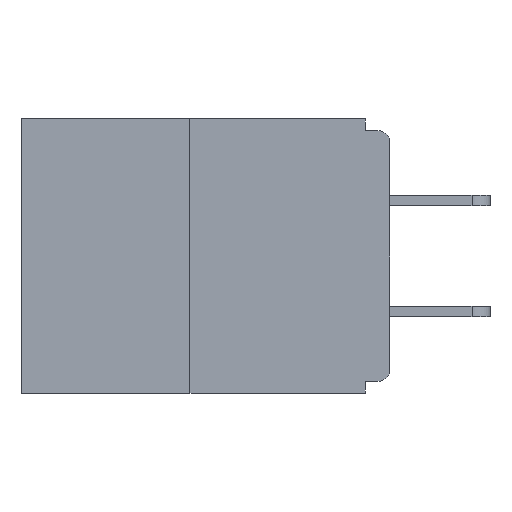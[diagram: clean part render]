
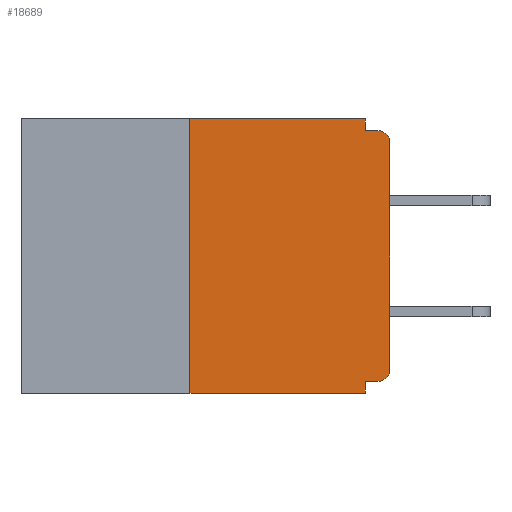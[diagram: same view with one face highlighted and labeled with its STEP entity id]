
A CAD part, left-side view. The second image highlights one B-rep face of the part: STEP entity #18689.
In plain terms, the highlighted planar face has unit normal (-1, 0, 0).
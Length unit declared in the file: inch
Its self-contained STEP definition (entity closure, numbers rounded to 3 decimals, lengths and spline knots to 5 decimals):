
#1026 = VERTEX_POINT ( 'NONE', #18729 ) ;
#1028 = CARTESIAN_POINT ( 'NONE',  ( 0., 0.46, 0. ) ) ;
#1231 = EDGE_CURVE ( 'NONE', #10391, #13205, #14252, .T. ) ;
#1282 = CARTESIAN_POINT ( 'NONE',  ( 0., 0.031, 0. ) ) ;
#1379 = EDGE_LOOP ( 'NONE', ( #12505, #6901, #14425, #8585, #7923, #14667, #17898, #1803, #16608, #10620 ) ) ;
#1416 = CARTESIAN_POINT ( 'NONE',  ( 0., 0., -0.015 ) ) ;
#1549 = CIRCLE ( 'NONE', #18769, 0.015 ) ;
#1803 = ORIENTED_EDGE ( 'NONE', *, *, #17479, .T. ) ;
#2152 = VECTOR ( 'NONE', #8442, 39.37008 ) ;
#2327 = CARTESIAN_POINT ( 'NONE',  ( 0., 0.031, -0.328 ) ) ;
#3012 = DIRECTION ( 'NONE',  ( 0., 0., -1. ) ) ;
#3296 = DIRECTION ( 'NONE',  ( 0., 1., 0. ) ) ;
#3542 = EDGE_CURVE ( 'NONE', #10391, #17923, #11056, .T. ) ;
#3973 = CARTESIAN_POINT ( 'NONE',  ( 0., 0.015, -0.313 ) ) ;
#4038 = DIRECTION ( 'NONE',  ( 0., 0., -1. ) ) ;
#4363 = LINE ( 'NONE', #1028, #18585 ) ;
#5464 = DIRECTION ( 'NONE',  ( 0., -1., 0. ) ) ;
#5690 = EDGE_CURVE ( 'NONE', #8635, #8324, #1549, .T. ) ;
#6554 = CARTESIAN_POINT ( 'NONE',  ( 0., 0.015, -0.03 ) ) ;
#6901 = ORIENTED_EDGE ( 'NONE', *, *, #3542, .F. ) ;
#6946 = DIRECTION ( 'NONE',  ( 0., 0., 1. ) ) ;
#7011 = CARTESIAN_POINT ( 'NONE',  ( 0., 0.25, 0. ) ) ;
#7147 = EDGE_CURVE ( 'NONE', #17923, #12711, #4363, .T. ) ;
#7442 = PLANE ( 'NONE',  #8067 ) ;
#7923 = ORIENTED_EDGE ( 'NONE', *, *, #11989, .F. ) ;
#8022 = DIRECTION ( 'NONE',  ( 0., 0., -1. ) ) ;
#8067 = AXIS2_PLACEMENT_3D ( 'NONE', #11747, #15289, #3012 ) ;
#8088 = LINE ( 'NONE', #19436, #18518 ) ;
#8324 = VERTEX_POINT ( 'NONE', #12617 ) ;
#8442 = DIRECTION ( 'NONE',  ( 0., -1., 0. ) ) ;
#8585 = ORIENTED_EDGE ( 'NONE', *, *, #10403, .F. ) ;
#8635 = VERTEX_POINT ( 'NONE', #10607 ) ;
#9167 = CARTESIAN_POINT ( 'NONE',  ( 0., 0.25, 0. ) ) ;
#9355 = VECTOR ( 'NONE', #3296, 39.37008 ) ;
#10145 = LINE ( 'NONE', #1282, #10378 ) ;
#10183 = EDGE_CURVE ( 'NONE', #12711, #17904, #10145, .T. ) ;
#10360 = VERTEX_POINT ( 'NONE', #2327 ) ;
#10378 = VECTOR ( 'NONE', #11878, 39.37008 ) ;
#10391 = VERTEX_POINT ( 'NONE', #18839 ) ;
#10403 = EDGE_CURVE ( 'NONE', #10360, #13205, #13717, .T. ) ;
#10540 = LINE ( 'NONE', #10839, #9355 ) ;
#10607 = CARTESIAN_POINT ( 'NONE',  ( 0., 0.015, -0.328 ) ) ;
#10620 = ORIENTED_EDGE ( 'NONE', *, *, #10183, .F. ) ;
#10839 = CARTESIAN_POINT ( 'NONE',  ( 0., 0., -0.328 ) ) ;
#11056 = LINE ( 'NONE', #7011, #18648 ) ;
#11747 = CARTESIAN_POINT ( 'NONE',  ( 0., 0.46, 0. ) ) ;
#11878 = DIRECTION ( 'NONE',  ( 0., 0., -1. ) ) ;
#11989 = EDGE_CURVE ( 'NONE', #8635, #10360, #10540, .T. ) ;
#12269 = VECTOR ( 'NONE', #14479, 39.37008 ) ;
#12505 = ORIENTED_EDGE ( 'NONE', *, *, #7147, .F. ) ;
#12617 = CARTESIAN_POINT ( 'NONE',  ( 0., 0., -0.313 ) ) ;
#12690 = CARTESIAN_POINT ( 'NONE',  ( 0., 0., -0.03 ) ) ;
#12711 = VERTEX_POINT ( 'NONE', #12980 ) ;
#12980 = CARTESIAN_POINT ( 'NONE',  ( 0., 0.031, 0. ) ) ;
#13205 = VERTEX_POINT ( 'NONE', #15621 ) ;
#13550 = DIRECTION ( 'NONE',  ( 0., 0., 1. ) ) ;
#13717 = LINE ( 'NONE', #19097, #12269 ) ;
#13831 = CIRCLE ( 'NONE', #19091, 0.015 ) ;
#14252 = LINE ( 'NONE', #17520, #2152 ) ;
#14315 = VERTEX_POINT ( 'NONE', #12690 ) ;
#14425 = ORIENTED_EDGE ( 'NONE', *, *, #1231, .T. ) ;
#14479 = DIRECTION ( 'NONE',  ( 0., 0., -1. ) ) ;
#14667 = ORIENTED_EDGE ( 'NONE', *, *, #5690, .T. ) ;
#14692 = EDGE_CURVE ( 'NONE', #8324, #14315, #8088, .T. ) ;
#15289 = DIRECTION ( 'NONE',  ( 1., 0., 0. ) ) ;
#15621 = CARTESIAN_POINT ( 'NONE',  ( 0., 0.031, -0.343 ) ) ;
#16423 = FACE_OUTER_BOUND ( 'NONE', #1379, .T. ) ;
#16608 = ORIENTED_EDGE ( 'NONE', *, *, #18651, .F. ) ;
#17479 = EDGE_CURVE ( 'NONE', #14315, #1026, #13831, .T. ) ;
#17520 = CARTESIAN_POINT ( 'NONE',  ( 0., 0.46, -0.343 ) ) ;
#17752 = DIRECTION ( 'NONE',  ( -1., 0., 0. ) ) ;
#17898 = ORIENTED_EDGE ( 'NONE', *, *, #14692, .T. ) ;
#17904 = VERTEX_POINT ( 'NONE', #19627 ) ;
#17923 = VERTEX_POINT ( 'NONE', #9167 ) ;
#18319 = VECTOR ( 'NONE', #19501, 39.37008 ) ;
#18518 = VECTOR ( 'NONE', #13550, 39.37008 ) ;
#18534 = LINE ( 'NONE', #1416, #18319 ) ;
#18543 = DIRECTION ( 'NONE',  ( -1., 0., 0. ) ) ;
#18585 = VECTOR ( 'NONE', #5464, 39.37008 ) ;
#18648 = VECTOR ( 'NONE', #6946, 39.37008 ) ;
#18651 = EDGE_CURVE ( 'NONE', #17904, #1026, #18534, .T. ) ;
#18689 = ADVANCED_FACE ( 'NONE', ( #16423 ), #7442, .F. ) ;
#18729 = CARTESIAN_POINT ( 'NONE',  ( 0., 0.015, -0.015 ) ) ;
#18769 = AXIS2_PLACEMENT_3D ( 'NONE', #3973, #17752, #4038 ) ;
#18839 = CARTESIAN_POINT ( 'NONE',  ( 0., 0.25, -0.343 ) ) ;
#19091 = AXIS2_PLACEMENT_3D ( 'NONE', #6554, #18543, #8022 ) ;
#19097 = CARTESIAN_POINT ( 'NONE',  ( 0., 0.031, -0.343 ) ) ;
#19436 = CARTESIAN_POINT ( 'NONE',  ( 0., 0., 0. ) ) ;
#19501 = DIRECTION ( 'NONE',  ( 0., -1., 0. ) ) ;
#19627 = CARTESIAN_POINT ( 'NONE',  ( 0., 0.031, -0.015 ) ) ;
